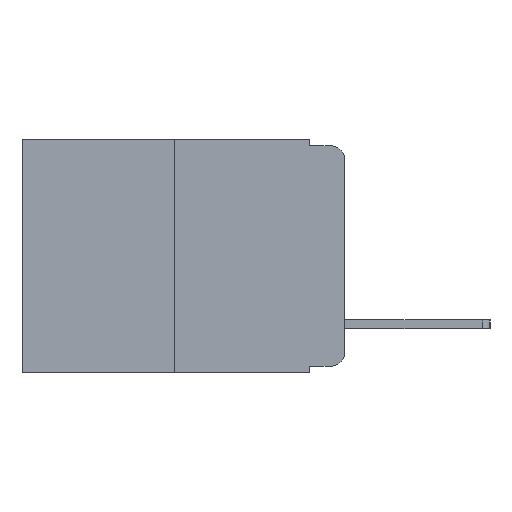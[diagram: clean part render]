
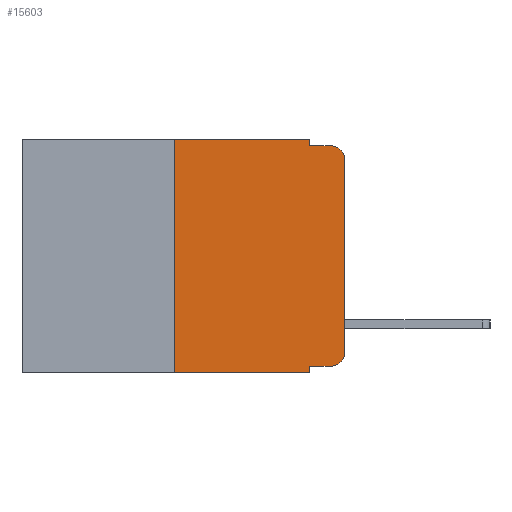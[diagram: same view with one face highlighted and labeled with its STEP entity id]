
A CAD part, left-side view. The second image highlights one B-rep face of the part: STEP entity #15603.
In plain terms, the highlighted planar face has unit normal (-1, 0, 0).
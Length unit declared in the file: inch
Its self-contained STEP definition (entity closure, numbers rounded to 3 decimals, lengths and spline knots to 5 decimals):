
#378 = CARTESIAN_POINT ( 'NONE',  ( 0., 0.051, 0. ) ) ;
#391 = LINE ( 'NONE', #8624, #19232 ) ;
#472 = DIRECTION ( 'NONE',  ( 0., 0., -1. ) ) ;
#593 = ORIENTED_EDGE ( 'NONE', *, *, #3238, .F. ) ;
#782 = EDGE_CURVE ( 'NONE', #11814, #17604, #391, .T. ) ;
#862 = CARTESIAN_POINT ( 'NONE',  ( 0., 0., -0.313 ) ) ;
#903 = EDGE_CURVE ( 'NONE', #10959, #11814, #4100, .T. ) ;
#996 = PLANE ( 'NONE',  #4006 ) ;
#1307 = CARTESIAN_POINT ( 'NONE',  ( 0., 0.02, -0.333 ) ) ;
#1821 = CARTESIAN_POINT ( 'NONE',  ( 0., 0.02, -0.03 ) ) ;
#2131 = EDGE_CURVE ( 'NONE', #17604, #18009, #2971, .T. ) ;
#2275 = VECTOR ( 'NONE', #2839, 39.37008 ) ;
#2388 = VECTOR ( 'NONE', #16931, 39.37008 ) ;
#2839 = DIRECTION ( 'NONE',  ( 0., -1., 0. ) ) ;
#2971 = LINE ( 'NONE', #17799, #7043 ) ;
#3238 = EDGE_CURVE ( 'NONE', #18009, #16912, #6016, .T. ) ;
#3438 = CARTESIAN_POINT ( 'NONE',  ( 0., 0., -0.03 ) ) ;
#3470 = DIRECTION ( 'NONE',  ( 0., 0., -1. ) ) ;
#4006 = AXIS2_PLACEMENT_3D ( 'NONE', #15988, #7401, #17378 ) ;
#4100 = LINE ( 'NONE', #10857, #11522 ) ;
#4257 = EDGE_CURVE ( 'NONE', #7869, #16912, #8592, .T. ) ;
#4819 = CIRCLE ( 'NONE', #12871, 0.02 ) ;
#4912 = LINE ( 'NONE', #378, #15612 ) ;
#5263 = EDGE_CURVE ( 'NONE', #13258, #7869, #8805, .T. ) ;
#5870 = CARTESIAN_POINT ( 'NONE',  ( 0., 0.02, -0.01 ) ) ;
#5901 = LINE ( 'NONE', #13229, #2275 ) ;
#5910 = CARTESIAN_POINT ( 'NONE',  ( 0., 0.051, -0.333 ) ) ;
#6016 = LINE ( 'NONE', #6905, #2388 ) ;
#6497 = CARTESIAN_POINT ( 'NONE',  ( 0., 0.25, 0. ) ) ;
#6733 = DIRECTION ( 'NONE',  ( 0., 0., -1. ) ) ;
#6905 = CARTESIAN_POINT ( 'NONE',  ( 0., 0.051, -0.01 ) ) ;
#6908 = ORIENTED_EDGE ( 'NONE', *, *, #5263, .T. ) ;
#6940 = EDGE_CURVE ( 'NONE', #10959, #8190, #5901, .T. ) ;
#7043 = VECTOR ( 'NONE', #6733, 39.37008 ) ;
#7401 = DIRECTION ( 'NONE',  ( 1., 0., 0. ) ) ;
#7646 = CARTESIAN_POINT ( 'NONE',  ( 0., 0., 0. ) ) ;
#7834 = VERTEX_POINT ( 'NONE', #10818 ) ;
#7869 = VERTEX_POINT ( 'NONE', #3438 ) ;
#8190 = VERTEX_POINT ( 'NONE', #12866 ) ;
#8461 = DIRECTION ( 'NONE',  ( -1., 0., 0. ) ) ;
#8592 = CIRCLE ( 'NONE', #13386, 0.02 ) ;
#8624 = CARTESIAN_POINT ( 'NONE',  ( 0., 0.473, 0. ) ) ;
#8692 = DIRECTION ( 'NONE',  ( 0., 0., 1. ) ) ;
#8805 = LINE ( 'NONE', #7646, #19210 ) ;
#8820 = EDGE_LOOP ( 'NONE', ( #6908, #15258, #593, #10739, #16032, #16928, #11837, #19076, #15571, #13752 ) ) ;
#9903 = DIRECTION ( 'NONE',  ( 0., -1., 0. ) ) ;
#10370 = VECTOR ( 'NONE', #17427, 39.37008 ) ;
#10739 = ORIENTED_EDGE ( 'NONE', *, *, #2131, .F. ) ;
#10818 = CARTESIAN_POINT ( 'NONE',  ( 0., 0.051, -0.333 ) ) ;
#10834 = LINE ( 'NONE', #5910, #10370 ) ;
#10857 = CARTESIAN_POINT ( 'NONE',  ( 0., 0.25, 0. ) ) ;
#10959 = VERTEX_POINT ( 'NONE', #17910 ) ;
#11522 = VECTOR ( 'NONE', #8692, 39.37008 ) ;
#11814 = VERTEX_POINT ( 'NONE', #6497 ) ;
#11837 = ORIENTED_EDGE ( 'NONE', *, *, #6940, .T. ) ;
#12366 = DIRECTION ( 'NONE',  ( -1., 0., 0. ) ) ;
#12866 = CARTESIAN_POINT ( 'NONE',  ( 0., 0.051, -0.343 ) ) ;
#12871 = AXIS2_PLACEMENT_3D ( 'NONE', #16964, #8461, #18365 ) ;
#13229 = CARTESIAN_POINT ( 'NONE',  ( 0., 0.473, -0.343 ) ) ;
#13258 = VERTEX_POINT ( 'NONE', #862 ) ;
#13386 = AXIS2_PLACEMENT_3D ( 'NONE', #1821, #12366, #3470 ) ;
#13752 = ORIENTED_EDGE ( 'NONE', *, *, #17252, .T. ) ;
#14410 = VERTEX_POINT ( 'NONE', #1307 ) ;
#15258 = ORIENTED_EDGE ( 'NONE', *, *, #4257, .T. ) ;
#15571 = ORIENTED_EDGE ( 'NONE', *, *, #18193, .T. ) ;
#15603 = ADVANCED_FACE ( 'NONE', ( #18208 ), #996, .F. ) ;
#15612 = VECTOR ( 'NONE', #472, 39.37008 ) ;
#15677 = CARTESIAN_POINT ( 'NONE',  ( 0., 0.051, -0.01 ) ) ;
#15988 = CARTESIAN_POINT ( 'NONE',  ( 0., 0.473, 0. ) ) ;
#16032 = ORIENTED_EDGE ( 'NONE', *, *, #782, .F. ) ;
#16191 = CARTESIAN_POINT ( 'NONE',  ( 0., 0.051, 0. ) ) ;
#16912 = VERTEX_POINT ( 'NONE', #5870 ) ;
#16928 = ORIENTED_EDGE ( 'NONE', *, *, #903, .F. ) ;
#16931 = DIRECTION ( 'NONE',  ( 0., -1., 0. ) ) ;
#16964 = CARTESIAN_POINT ( 'NONE',  ( 0., 0.02, -0.313 ) ) ;
#17252 = EDGE_CURVE ( 'NONE', #14410, #13258, #4819, .T. ) ;
#17378 = DIRECTION ( 'NONE',  ( 0., 0., -1. ) ) ;
#17427 = DIRECTION ( 'NONE',  ( 0., -1., 0. ) ) ;
#17594 = DIRECTION ( 'NONE',  ( 0., 0., 1. ) ) ;
#17604 = VERTEX_POINT ( 'NONE', #16191 ) ;
#17799 = CARTESIAN_POINT ( 'NONE',  ( 0., 0.051, 0. ) ) ;
#17910 = CARTESIAN_POINT ( 'NONE',  ( 0., 0.25, -0.343 ) ) ;
#18009 = VERTEX_POINT ( 'NONE', #15677 ) ;
#18193 = EDGE_CURVE ( 'NONE', #7834, #14410, #10834, .T. ) ;
#18208 = FACE_OUTER_BOUND ( 'NONE', #8820, .T. ) ;
#18365 = DIRECTION ( 'NONE',  ( 0., 0., -1. ) ) ;
#19076 = ORIENTED_EDGE ( 'NONE', *, *, #19137, .F. ) ;
#19137 = EDGE_CURVE ( 'NONE', #7834, #8190, #4912, .T. ) ;
#19210 = VECTOR ( 'NONE', #17594, 39.37008 ) ;
#19232 = VECTOR ( 'NONE', #9903, 39.37008 ) ;
